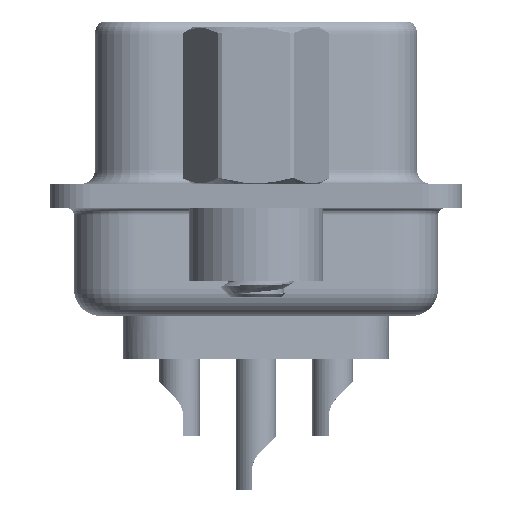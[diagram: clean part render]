
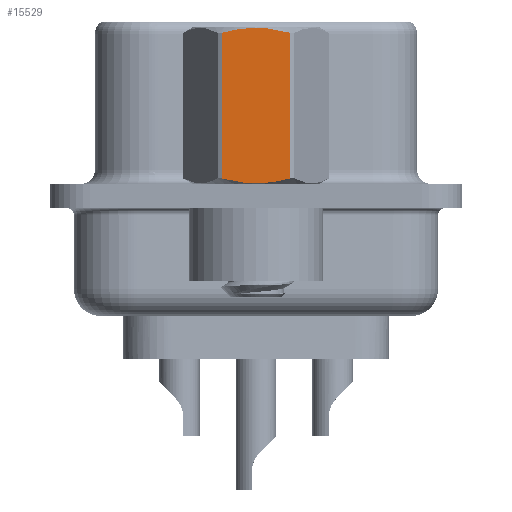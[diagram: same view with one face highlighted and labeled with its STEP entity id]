
A CAD part, left-side view. The second image highlights one B-rep face of the part: STEP entity #15529.
In plain terms, the highlighted planar face has unit normal (-1, 0, 0).
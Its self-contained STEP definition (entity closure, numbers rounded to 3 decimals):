
#186 = VERTEX_POINT ( 'NONE', #1496 ) ;
#882 = ORIENTED_EDGE ( 'NONE', *, *, #4998, .T. ) ;
#1050 = CARTESIAN_POINT ( 'NONE',  ( -2.381, -1.273, 3.792 ) ) ;
#1259 = CARTESIAN_POINT ( 'NONE',  ( -2.381, 1.065, 0.596 ) ) ;
#1363 = DIRECTION ( 'NONE',  ( -1., 0., 0. ) ) ;
#1496 = CARTESIAN_POINT ( 'NONE',  ( -2.381, -1.273, 6.048 ) ) ;
#1973 = CARTESIAN_POINT ( 'NONE',  ( -2.381, -1.273, 6.048 ) ) ;
#2190 = CARTESIAN_POINT ( 'NONE',  ( -2.381, 1.273, 6.048 ) ) ;
#4139 = PLANE ( 'NONE',  #35534 ) ;
#4148 = CARTESIAN_POINT ( 'NONE',  ( -2.381, 1.273, 0.652 ) ) ;
#4655 = VERTEX_POINT ( 'NONE', #36453 ) ;
#4830 = CARTESIAN_POINT ( 'NONE',  ( -2.381, -1.066, 6.104 ) ) ;
#4998 = EDGE_CURVE ( 'NONE', #4655, #29264, #22175, .T. ) ;
#5511 = B_SPLINE_CURVE_WITH_KNOTS ( 'NONE', 3,
 ( #1973, #4830, #10699, #30759, #13601, #33668, #16459, #36580, #19370, #2190 ),
 .UNSPECIFIED., .F., .F.,
 ( 4, 2, 2, 2, 4 ),
 ( 0.001, 0.002, 0.002, 0.003, 0.004 ),
 .UNSPECIFIED. ) ;
#5669 = EDGE_CURVE ( 'NONE', #29264, #37048, #27196, .T. ) ;
#6295 = CARTESIAN_POINT ( 'NONE',  ( -2.381, 1.273, 3.792 ) ) ;
#7021 = CARTESIAN_POINT ( 'NONE',  ( -2.381, 0.428, 0.485 ) ) ;
#9581 = ORIENTED_EDGE ( 'NONE', *, *, #19593, .T. ) ;
#9875 = CARTESIAN_POINT ( 'NONE',  ( -2.381, -0.215, 0.468 ) ) ;
#10608 = CARTESIAN_POINT ( 'NONE',  ( -2.381, 1.273, 0.652 ) ) ;
#10699 = CARTESIAN_POINT ( 'NONE',  ( -2.381, -0.858, 6.15 ) ) ;
#12018 = VECTOR ( 'NONE', #18198, 1000. ) ;
#12763 = CARTESIAN_POINT ( 'NONE',  ( -2.381, 1.375, -3.75 ) ) ;
#12769 = CARTESIAN_POINT ( 'NONE',  ( -2.381, -0.858, 0.55 ) ) ;
#13601 = CARTESIAN_POINT ( 'NONE',  ( -2.381, -0.215, 6.232 ) ) ;
#15529 = ADVANCED_FACE ( 'NONE', ( #21051 ), #4139, .T. ) ;
#15646 = CARTESIAN_POINT ( 'NONE',  ( -2.381, -1.273, 0.652 ) ) ;
#16459 = CARTESIAN_POINT ( 'NONE',  ( -2.381, 0.428, 6.215 ) ) ;
#16710 = LINE ( 'NONE', #1050, #12018 ) ;
#16809 = EDGE_CURVE ( 'NONE', #186, #4655, #5511, .T. ) ;
#17593 = ORIENTED_EDGE ( 'NONE', *, *, #16809, .T. ) ;
#18198 = DIRECTION ( 'NONE',  ( 0., 0., 1. ) ) ;
#18407 = CARTESIAN_POINT ( 'NONE',  ( -2.381, 0.853, 0.549 ) ) ;
#19370 = CARTESIAN_POINT ( 'NONE',  ( -2.381, 1.065, 6.104 ) ) ;
#19593 = EDGE_CURVE ( 'NONE', #37048, #186, #16710, .T. ) ;
#20146 = EDGE_LOOP ( 'NONE', ( #26922, #9581, #17593, #882 ) ) ;
#20383 = VECTOR ( 'NONE', #35171, 1000. ) ;
#21051 = FACE_OUTER_BOUND ( 'NONE', #20146, .T. ) ;
#21425 = DIRECTION ( 'NONE',  ( 0., -1., 0. ) ) ;
#22175 = LINE ( 'NONE', #6295, #20383 ) ;
#26922 = ORIENTED_EDGE ( 'NONE', *, *, #5669, .T. ) ;
#27072 = CARTESIAN_POINT ( 'NONE',  ( -2.381, 0.215, 0.468 ) ) ;
#27196 = B_SPLINE_CURVE_WITH_KNOTS ( 'NONE', 3,
 ( #4148, #1259, #18407, #7021, #27072, #9875, #29919, #12769, #32836, #15646 ),
 .UNSPECIFIED., .F., .F.,
 ( 4, 2, 2, 2, 4 ),
 ( 0.003, 0.003, 0.004, 0.004, 0.005 ),
 .UNSPECIFIED. ) ;
#29264 = VERTEX_POINT ( 'NONE', #10608 ) ;
#29919 = CARTESIAN_POINT ( 'NONE',  ( -2.381, -0.432, 0.485 ) ) ;
#30759 = CARTESIAN_POINT ( 'NONE',  ( -2.381, -0.432, 6.215 ) ) ;
#32836 = CARTESIAN_POINT ( 'NONE',  ( -2.381, -1.066, 0.596 ) ) ;
#33668 = CARTESIAN_POINT ( 'NONE',  ( -2.381, 0.215, 6.232 ) ) ;
#34985 = CARTESIAN_POINT ( 'NONE',  ( -2.381, -1.273, 0.652 ) ) ;
#35171 = DIRECTION ( 'NONE',  ( 0., 0., -1. ) ) ;
#35534 = AXIS2_PLACEMENT_3D ( 'NONE', #12763, #1363, #21425 ) ;
#36453 = CARTESIAN_POINT ( 'NONE',  ( -2.381, 1.273, 6.048 ) ) ;
#36580 = CARTESIAN_POINT ( 'NONE',  ( -2.381, 0.853, 6.151 ) ) ;
#37048 = VERTEX_POINT ( 'NONE', #34985 ) ;
